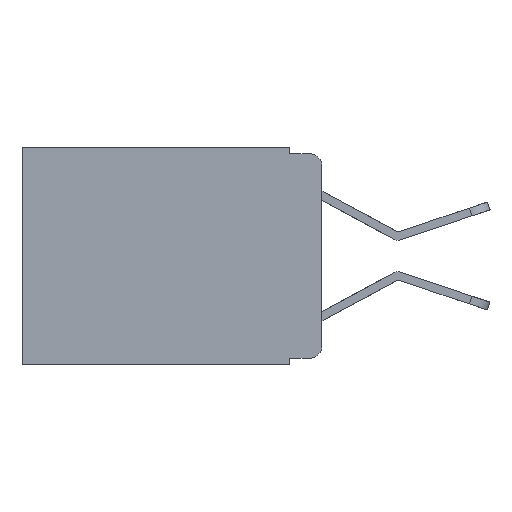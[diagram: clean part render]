
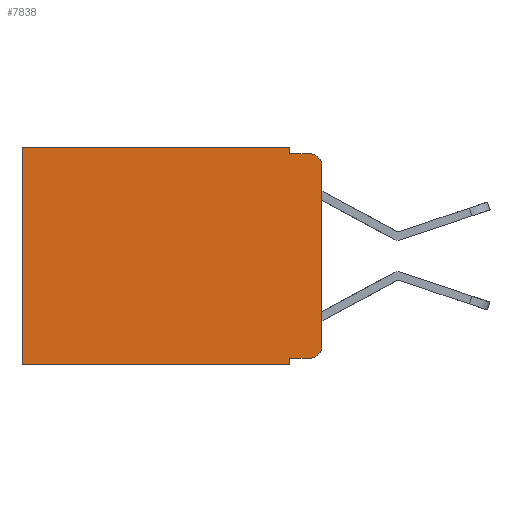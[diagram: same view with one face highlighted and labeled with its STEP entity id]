
A CAD part, left-side view. The second image highlights one B-rep face of the part: STEP entity #7838.
In plain terms, the highlighted planar face has unit normal (-1, 0, 0).
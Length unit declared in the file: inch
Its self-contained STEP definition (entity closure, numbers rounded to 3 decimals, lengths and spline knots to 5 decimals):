
#714 = VECTOR ( 'NONE', #7091, 39.37008 ) ;
#810 = EDGE_CURVE ( 'NONE', #16668, #18782, #8799, .T. ) ;
#842 = CARTESIAN_POINT ( 'NONE',  ( 0.298, 0.473, -0.343 ) ) ;
#1110 = CARTESIAN_POINT ( 'NONE',  ( 0.298, 0.473, 0. ) ) ;
#1301 = VERTEX_POINT ( 'NONE', #15442 ) ;
#1556 = CARTESIAN_POINT ( 'NONE',  ( 0.298, 0.02, -0.03 ) ) ;
#1658 = VERTEX_POINT ( 'NONE', #842 ) ;
#1843 = EDGE_CURVE ( 'NONE', #9738, #1658, #18651, .T. ) ;
#2177 = CARTESIAN_POINT ( 'NONE',  ( 0.298, 0., -0.313 ) ) ;
#2380 = AXIS2_PLACEMENT_3D ( 'NONE', #18653, #10433, #11709 ) ;
#2566 = LINE ( 'NONE', #6511, #17402 ) ;
#2893 = EDGE_CURVE ( 'NONE', #13617, #17460, #12689, .T. ) ;
#3395 = DIRECTION ( 'NONE',  ( 0., 0., -1. ) ) ;
#3778 = ORIENTED_EDGE ( 'NONE', *, *, #810, .F. ) ;
#3921 = EDGE_CURVE ( 'NONE', #17460, #11540, #4822, .T. ) ;
#3924 = CARTESIAN_POINT ( 'NONE',  ( 0.298, 0.473, 0. ) ) ;
#3983 = CARTESIAN_POINT ( 'NONE',  ( 0.298, 0., -0.343 ) ) ;
#4187 = CARTESIAN_POINT ( 'NONE',  ( 0.298, 0.051, -0.333 ) ) ;
#4312 = CARTESIAN_POINT ( 'NONE',  ( 0.298, 0.02, -0.313 ) ) ;
#4822 = LINE ( 'NONE', #5091, #714 ) ;
#5091 = CARTESIAN_POINT ( 'NONE',  ( 0.298, 0.051, -0.01 ) ) ;
#5094 = CIRCLE ( 'NONE', #9903, 0.02 ) ;
#5402 = CARTESIAN_POINT ( 'NONE',  ( 0.298, 0.051, -0.333 ) ) ;
#5415 = DIRECTION ( 'NONE',  ( 0., 1., 0. ) ) ;
#5820 = DIRECTION ( 'NONE',  ( 0., 0., -1. ) ) ;
#5893 = VERTEX_POINT ( 'NONE', #2177 ) ;
#5924 = EDGE_CURVE ( 'NONE', #1301, #11540, #5094, .T. ) ;
#6322 = DIRECTION ( 'NONE',  ( 0., 0., -1. ) ) ;
#6511 = CARTESIAN_POINT ( 'NONE',  ( 0.298, 0., 0. ) ) ;
#6594 = LINE ( 'NONE', #3983, #7069 ) ;
#6619 = CARTESIAN_POINT ( 'NONE',  ( 0.298, 0.051, 0. ) ) ;
#6883 = DIRECTION ( 'NONE',  ( 0., -1., 0. ) ) ;
#7000 = DIRECTION ( 'NONE',  ( 0., 0., -1. ) ) ;
#7033 = LINE ( 'NONE', #7392, #14086 ) ;
#7069 = VECTOR ( 'NONE', #5415, 39.37008 ) ;
#7091 = DIRECTION ( 'NONE',  ( 0., -1., 0. ) ) ;
#7392 = CARTESIAN_POINT ( 'NONE',  ( 0.298, 0., 0. ) ) ;
#7563 = ORIENTED_EDGE ( 'NONE', *, *, #9238, .T. ) ;
#7597 = DIRECTION ( 'NONE',  ( 0., 0., -1. ) ) ;
#7600 = DIRECTION ( 'NONE',  ( -1., 0., 0. ) ) ;
#7838 = ADVANCED_FACE ( 'NONE', ( #12167 ), #15171, .F. ) ;
#7881 = AXIS2_PLACEMENT_3D ( 'NONE', #4312, #14312, #5820 ) ;
#8409 = EDGE_CURVE ( 'NONE', #18782, #1658, #6594, .T. ) ;
#8799 = LINE ( 'NONE', #11390, #12533 ) ;
#8841 = DIRECTION ( 'NONE',  ( 0., 1., 0. ) ) ;
#8845 = CIRCLE ( 'NONE', #7881, 0.02 ) ;
#8854 = EDGE_CURVE ( 'NONE', #1301, #5893, #2566, .T. ) ;
#8920 = DIRECTION ( 'NONE',  ( 0., 0., -1. ) ) ;
#8944 = VECTOR ( 'NONE', #7000, 39.37008 ) ;
#8952 = ORIENTED_EDGE ( 'NONE', *, *, #17667, .T. ) ;
#9238 = EDGE_CURVE ( 'NONE', #13617, #9738, #7033, .T. ) ;
#9359 = CARTESIAN_POINT ( 'NONE',  ( 0.298, 0.051, -0.343 ) ) ;
#9738 = VERTEX_POINT ( 'NONE', #3924 ) ;
#9780 = ORIENTED_EDGE ( 'NONE', *, *, #8854, .F. ) ;
#9903 = AXIS2_PLACEMENT_3D ( 'NONE', #1556, #7600, #7597 ) ;
#9979 = ORIENTED_EDGE ( 'NONE', *, *, #2893, .F. ) ;
#10341 = VECTOR ( 'NONE', #6883, 39.37008 ) ;
#10433 = DIRECTION ( 'NONE',  ( 1., 0., 0. ) ) ;
#11390 = CARTESIAN_POINT ( 'NONE',  ( 0.298, 0.051, 0. ) ) ;
#11411 = VERTEX_POINT ( 'NONE', #12178 ) ;
#11540 = VERTEX_POINT ( 'NONE', #16718 ) ;
#11709 = DIRECTION ( 'NONE',  ( 0., 0., -1. ) ) ;
#12008 = ORIENTED_EDGE ( 'NONE', *, *, #3921, .F. ) ;
#12155 = ORIENTED_EDGE ( 'NONE', *, *, #16722, .T. ) ;
#12167 = FACE_OUTER_BOUND ( 'NONE', #15776, .T. ) ;
#12178 = CARTESIAN_POINT ( 'NONE',  ( 0.298, 0.02, -0.333 ) ) ;
#12211 = ORIENTED_EDGE ( 'NONE', *, *, #1843, .T. ) ;
#12533 = VECTOR ( 'NONE', #6322, 39.37008 ) ;
#12689 = LINE ( 'NONE', #16547, #8944 ) ;
#13116 = ORIENTED_EDGE ( 'NONE', *, *, #8409, .F. ) ;
#13617 = VERTEX_POINT ( 'NONE', #6619 ) ;
#14066 = LINE ( 'NONE', #5402, #10341 ) ;
#14086 = VECTOR ( 'NONE', #8841, 39.37008 ) ;
#14312 = DIRECTION ( 'NONE',  ( -1., 0., 0. ) ) ;
#15171 = PLANE ( 'NONE',  #2380 ) ;
#15286 = ORIENTED_EDGE ( 'NONE', *, *, #5924, .T. ) ;
#15331 = VECTOR ( 'NONE', #3395, 39.37008 ) ;
#15442 = CARTESIAN_POINT ( 'NONE',  ( 0.298, 0., -0.03 ) ) ;
#15776 = EDGE_LOOP ( 'NONE', ( #9780, #15286, #12008, #9979, #7563, #12211, #13116, #3778, #8952, #12155 ) ) ;
#16257 = CARTESIAN_POINT ( 'NONE',  ( 0.298, 0.051, -0.01 ) ) ;
#16547 = CARTESIAN_POINT ( 'NONE',  ( 0.298, 0.051, 0. ) ) ;
#16668 = VERTEX_POINT ( 'NONE', #4187 ) ;
#16718 = CARTESIAN_POINT ( 'NONE',  ( 0.298, 0.02, -0.01 ) ) ;
#16722 = EDGE_CURVE ( 'NONE', #11411, #5893, #8845, .T. ) ;
#17402 = VECTOR ( 'NONE', #8920, 39.37008 ) ;
#17460 = VERTEX_POINT ( 'NONE', #16257 ) ;
#17667 = EDGE_CURVE ( 'NONE', #16668, #11411, #14066, .T. ) ;
#18651 = LINE ( 'NONE', #1110, #15331 ) ;
#18653 = CARTESIAN_POINT ( 'NONE',  ( 0.298, 0., 0. ) ) ;
#18782 = VERTEX_POINT ( 'NONE', #9359 ) ;
